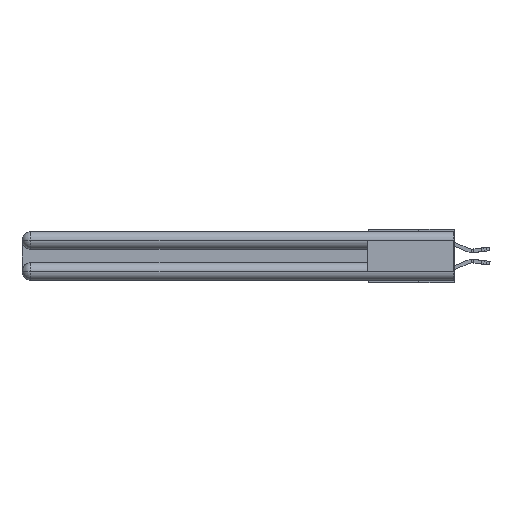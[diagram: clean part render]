
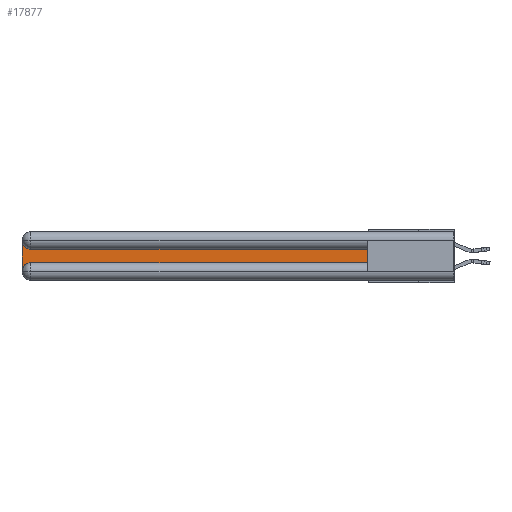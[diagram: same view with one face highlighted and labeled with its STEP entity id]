
A CAD part, left-side view. The second image highlights one B-rep face of the part: STEP entity #17877.
In plain terms, the highlighted planar face has unit normal (-1, 0, 0).
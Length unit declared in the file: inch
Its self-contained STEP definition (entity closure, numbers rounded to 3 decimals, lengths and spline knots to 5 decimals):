
#55 = ORIENTED_EDGE ( 'NONE', *, *, #16282, .T. ) ;
#515 = DIRECTION ( 'NONE',  ( 0., 0., -1. ) ) ;
#1020 = VERTEX_POINT ( 'NONE', #24776 ) ;
#1611 = LINE ( 'NONE', #23030, #18453 ) ;
#2058 = CIRCLE ( 'NONE', #18650, 0.06 ) ;
#3775 = EDGE_CURVE ( 'NONE', #18939, #16356, #4582, .T. ) ;
#3830 = VECTOR ( 'NONE', #6371, 39.37008 ) ;
#4582 = LINE ( 'NONE', #8621, #3830 ) ;
#6135 = DIRECTION ( 'NONE',  ( 1., 0., 0. ) ) ;
#6254 = CARTESIAN_POINT ( 'NONE',  ( 0.075, 3., -0.2175 ) ) ;
#6371 = DIRECTION ( 'NONE',  ( 0., -1., 0. ) ) ;
#6517 = ORIENTED_EDGE ( 'NONE', *, *, #10989, .T. ) ;
#7809 = CARTESIAN_POINT ( 'NONE',  ( 0.075, 2.94, -0.0625 ) ) ;
#8621 = CARTESIAN_POINT ( 'NONE',  ( 0.075, 0.6, -0.2175 ) ) ;
#8646 = CARTESIAN_POINT ( 'NONE',  ( 0.075, 2.94, -0.1225 ) ) ;
#9234 = VERTEX_POINT ( 'NONE', #14320 ) ;
#10381 = CARTESIAN_POINT ( 'NONE',  ( 0.075, 0.6, -0.2175 ) ) ;
#10929 = CARTESIAN_POINT ( 'NONE',  ( 0.075, 2.94, -0.2775 ) ) ;
#10989 = EDGE_CURVE ( 'NONE', #9234, #1020, #19853, .T. ) ;
#11426 = CIRCLE ( 'NONE', #24678, 0.06 ) ;
#11597 = AXIS2_PLACEMENT_3D ( 'NONE', #22777, #30559, #27891 ) ;
#12210 = EDGE_CURVE ( 'NONE', #1020, #18939, #2058, .T. ) ;
#12661 = ORIENTED_EDGE ( 'NONE', *, *, #26615, .T. ) ;
#12872 = FACE_OUTER_BOUND ( 'NONE', #26370, .T. ) ;
#13407 = DIRECTION ( 'NONE',  ( 0., 0., -1. ) ) ;
#13995 = ORIENTED_EDGE ( 'NONE', *, *, #12210, .T. ) ;
#14320 = CARTESIAN_POINT ( 'NONE',  ( 0.075, 3., -0.0625 ) ) ;
#14422 = VECTOR ( 'NONE', #15501, 39.37008 ) ;
#15501 = DIRECTION ( 'NONE',  ( 0., 1., 0. ) ) ;
#16282 = EDGE_CURVE ( 'NONE', #30009, #19457, #26262, .T. ) ;
#16356 = VERTEX_POINT ( 'NONE', #10381 ) ;
#17877 = ADVANCED_FACE ( 'NONE', ( #12872 ), #30256, .F. ) ;
#18453 = VECTOR ( 'NONE', #30394, 39.37008 ) ;
#18650 = AXIS2_PLACEMENT_3D ( 'NONE', #10929, #6135, #13407 ) ;
#18939 = VERTEX_POINT ( 'NONE', #19347 ) ;
#19009 = ORIENTED_EDGE ( 'NONE', *, *, #19031, .T. ) ;
#19031 = EDGE_CURVE ( 'NONE', #19457, #9234, #11426, .T. ) ;
#19347 = CARTESIAN_POINT ( 'NONE',  ( 0.075, 2.94, -0.2175 ) ) ;
#19457 = VERTEX_POINT ( 'NONE', #8646 ) ;
#19853 = LINE ( 'NONE', #6254, #20666 ) ;
#20666 = VECTOR ( 'NONE', #21009, 39.37008 ) ;
#21009 = DIRECTION ( 'NONE',  ( 0., 0., -1. ) ) ;
#22020 = DIRECTION ( 'NONE',  ( 1., 0., 0. ) ) ;
#22777 = CARTESIAN_POINT ( 'NONE',  ( 0.075, 3., -0.1225 ) ) ;
#23030 = CARTESIAN_POINT ( 'NONE',  ( 0.075, 0.6, -0.2175 ) ) ;
#24678 = AXIS2_PLACEMENT_3D ( 'NONE', #7809, #22020, #515 ) ;
#24776 = CARTESIAN_POINT ( 'NONE',  ( 0.075, 3., -0.2775 ) ) ;
#26262 = LINE ( 'NONE', #30144, #14422 ) ;
#26370 = EDGE_LOOP ( 'NONE', ( #55, #19009, #6517, #13995, #27422, #12661 ) ) ;
#26615 = EDGE_CURVE ( 'NONE', #16356, #30009, #1611, .T. ) ;
#27422 = ORIENTED_EDGE ( 'NONE', *, *, #3775, .T. ) ;
#27891 = DIRECTION ( 'NONE',  ( 0., 0., -1. ) ) ;
#28485 = CARTESIAN_POINT ( 'NONE',  ( 0.075, 0.6, -0.1225 ) ) ;
#30009 = VERTEX_POINT ( 'NONE', #28485 ) ;
#30144 = CARTESIAN_POINT ( 'NONE',  ( 0.075, 0.6, -0.1225 ) ) ;
#30256 = PLANE ( 'NONE',  #11597 ) ;
#30394 = DIRECTION ( 'NONE',  ( 0., 0., 1. ) ) ;
#30559 = DIRECTION ( 'NONE',  ( 1., 0., 0. ) ) ;
